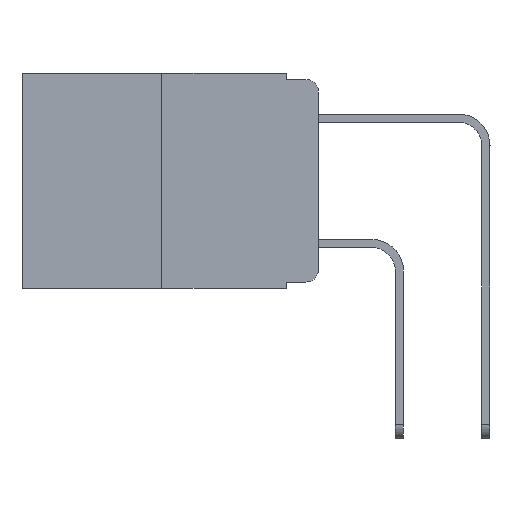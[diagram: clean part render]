
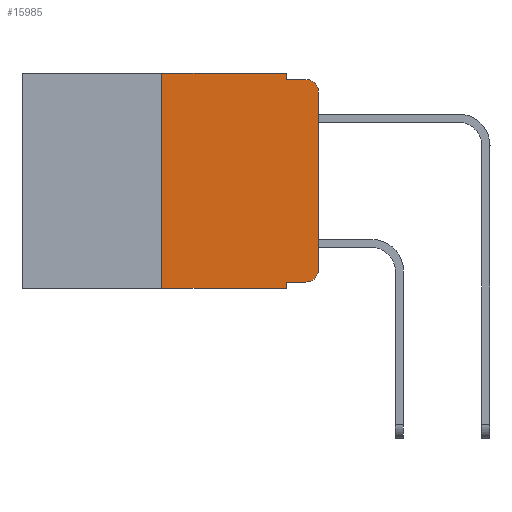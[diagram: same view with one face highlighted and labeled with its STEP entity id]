
A CAD part, left-side view. The second image highlights one B-rep face of the part: STEP entity #15985.
In plain terms, the highlighted planar face has unit normal (-1, 0, 0).
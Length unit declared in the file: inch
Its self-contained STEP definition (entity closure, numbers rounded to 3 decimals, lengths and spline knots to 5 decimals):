
#83 = VECTOR ( 'NONE', #18770, 39.37008 ) ;
#1247 = DIRECTION ( 'NONE',  ( 0., -1., 0. ) ) ;
#1356 = EDGE_CURVE ( 'NONE', #2703, #6175, #15612, .T. ) ;
#1465 = PLANE ( 'NONE',  #12127 ) ;
#1595 = EDGE_CURVE ( 'NONE', #11522, #7091, #17260, .T. ) ;
#1651 = CARTESIAN_POINT ( 'NONE',  ( 0., 0.051, -0.01 ) ) ;
#1999 = EDGE_CURVE ( 'NONE', #16640, #8751, #3684, .T. ) ;
#2165 = ORIENTED_EDGE ( 'NONE', *, *, #15334, .T. ) ;
#2244 = CARTESIAN_POINT ( 'NONE',  ( 0., 0., 0. ) ) ;
#2339 = ORIENTED_EDGE ( 'NONE', *, *, #1595, .F. ) ;
#2703 = VERTEX_POINT ( 'NONE', #9197 ) ;
#3211 = ORIENTED_EDGE ( 'NONE', *, *, #10394, .F. ) ;
#3255 = AXIS2_PLACEMENT_3D ( 'NONE', #13335, #4582, #4142 ) ;
#3684 = CIRCLE ( 'NONE', #13713, 0.02 ) ;
#3781 = VECTOR ( 'NONE', #10715, 39.37008 ) ;
#3788 = LINE ( 'NONE', #1651, #3781 ) ;
#3807 = DIRECTION ( 'NONE',  ( 0., -1., 0. ) ) ;
#3829 = DIRECTION ( 'NONE',  ( 0., 0., -1. ) ) ;
#4125 = FACE_OUTER_BOUND ( 'NONE', #10324, .T. ) ;
#4142 = DIRECTION ( 'NONE',  ( 0., 0., -1. ) ) ;
#4145 = LINE ( 'NONE', #5860, #5555 ) ;
#4582 = DIRECTION ( 'NONE',  ( -1., 0., 0. ) ) ;
#4693 = LINE ( 'NONE', #7018, #19431 ) ;
#5419 = EDGE_CURVE ( 'NONE', #13062, #10968, #4693, .T. ) ;
#5555 = VECTOR ( 'NONE', #10460, 39.37008 ) ;
#5860 = CARTESIAN_POINT ( 'NONE',  ( 0., 0.051, -0.333 ) ) ;
#6067 = CARTESIAN_POINT ( 'NONE',  ( 0., 0.473, 0. ) ) ;
#6175 = VERTEX_POINT ( 'NONE', #8350 ) ;
#6269 = CIRCLE ( 'NONE', #3255, 0.02 ) ;
#6713 = LINE ( 'NONE', #15894, #13593 ) ;
#7018 = CARTESIAN_POINT ( 'NONE',  ( 0., 0.051, 0. ) ) ;
#7091 = VERTEX_POINT ( 'NONE', #19021 ) ;
#7314 = DIRECTION ( 'NONE',  ( 0., 0., -1. ) ) ;
#7614 = DIRECTION ( 'NONE',  ( 0., 0., -1. ) ) ;
#7619 = DIRECTION ( 'NONE',  ( 0., 0., -1. ) ) ;
#7679 = DIRECTION ( 'NONE',  ( -1., 0., 0. ) ) ;
#7975 = VERTEX_POINT ( 'NONE', #14895 ) ;
#8350 = CARTESIAN_POINT ( 'NONE',  ( 0., 0.25, 0. ) ) ;
#8414 = CARTESIAN_POINT ( 'NONE',  ( 0., 0.051, 0. ) ) ;
#8751 = VERTEX_POINT ( 'NONE', #10930 ) ;
#9197 = CARTESIAN_POINT ( 'NONE',  ( 0., 0.25, -0.343 ) ) ;
#9315 = CARTESIAN_POINT ( 'NONE',  ( 0., 0.051, -0.01 ) ) ;
#9474 = ORIENTED_EDGE ( 'NONE', *, *, #10550, .T. ) ;
#9818 = ORIENTED_EDGE ( 'NONE', *, *, #16321, .T. ) ;
#10324 = EDGE_LOOP ( 'NONE', ( #9818, #11984, #10489, #15270, #3211, #14502, #9474, #2339, #2165, #16819 ) ) ;
#10394 = EDGE_CURVE ( 'NONE', #6175, #13062, #16227, .T. ) ;
#10460 = DIRECTION ( 'NONE',  ( 0., -1., 0. ) ) ;
#10489 = ORIENTED_EDGE ( 'NONE', *, *, #12215, .F. ) ;
#10550 = EDGE_CURVE ( 'NONE', #2703, #7091, #6713, .T. ) ;
#10715 = DIRECTION ( 'NONE',  ( 0., -1., 0. ) ) ;
#10930 = CARTESIAN_POINT ( 'NONE',  ( 0., 0., -0.313 ) ) ;
#10968 = VERTEX_POINT ( 'NONE', #9315 ) ;
#11522 = VERTEX_POINT ( 'NONE', #16805 ) ;
#11984 = ORIENTED_EDGE ( 'NONE', *, *, #15957, .T. ) ;
#12042 = DIRECTION ( 'NONE',  ( 1., 0., 0. ) ) ;
#12127 = AXIS2_PLACEMENT_3D ( 'NONE', #16720, #12042, #7614 ) ;
#12215 = EDGE_CURVE ( 'NONE', #10968, #7975, #3788, .T. ) ;
#12397 = CARTESIAN_POINT ( 'NONE',  ( 0., 0.25, 0. ) ) ;
#13062 = VERTEX_POINT ( 'NONE', #8414 ) ;
#13335 = CARTESIAN_POINT ( 'NONE',  ( 0., 0.02, -0.03 ) ) ;
#13593 = VECTOR ( 'NONE', #3807, 39.37008 ) ;
#13713 = AXIS2_PLACEMENT_3D ( 'NONE', #16724, #7679, #7619 ) ;
#13939 = DIRECTION ( 'NONE',  ( 0., 0., 1. ) ) ;
#14413 = VERTEX_POINT ( 'NONE', #18862 ) ;
#14502 = ORIENTED_EDGE ( 'NONE', *, *, #1356, .F. ) ;
#14895 = CARTESIAN_POINT ( 'NONE',  ( 0., 0.02, -0.01 ) ) ;
#15270 = ORIENTED_EDGE ( 'NONE', *, *, #5419, .F. ) ;
#15334 = EDGE_CURVE ( 'NONE', #11522, #16640, #4145, .T. ) ;
#15612 = LINE ( 'NONE', #12397, #16317 ) ;
#15894 = CARTESIAN_POINT ( 'NONE',  ( 0., 0.473, -0.343 ) ) ;
#15957 = EDGE_CURVE ( 'NONE', #14413, #7975, #6269, .T. ) ;
#15985 = ADVANCED_FACE ( 'NONE', ( #4125 ), #1465, .F. ) ;
#16227 = LINE ( 'NONE', #6067, #17900 ) ;
#16279 = CARTESIAN_POINT ( 'NONE',  ( 0., 0.051, 0. ) ) ;
#16317 = VECTOR ( 'NONE', #13939, 39.37008 ) ;
#16321 = EDGE_CURVE ( 'NONE', #8751, #14413, #16719, .T. ) ;
#16640 = VERTEX_POINT ( 'NONE', #18238 ) ;
#16719 = LINE ( 'NONE', #2244, #83 ) ;
#16720 = CARTESIAN_POINT ( 'NONE',  ( 0., 0.473, 0. ) ) ;
#16724 = CARTESIAN_POINT ( 'NONE',  ( 0., 0.02, -0.313 ) ) ;
#16805 = CARTESIAN_POINT ( 'NONE',  ( 0., 0.051, -0.333 ) ) ;
#16819 = ORIENTED_EDGE ( 'NONE', *, *, #1999, .T. ) ;
#17260 = LINE ( 'NONE', #16279, #18924 ) ;
#17900 = VECTOR ( 'NONE', #1247, 39.37008 ) ;
#18238 = CARTESIAN_POINT ( 'NONE',  ( 0., 0.02, -0.333 ) ) ;
#18770 = DIRECTION ( 'NONE',  ( 0., 0., 1. ) ) ;
#18862 = CARTESIAN_POINT ( 'NONE',  ( 0., 0., -0.03 ) ) ;
#18924 = VECTOR ( 'NONE', #7314, 39.37008 ) ;
#19021 = CARTESIAN_POINT ( 'NONE',  ( 0., 0.051, -0.343 ) ) ;
#19431 = VECTOR ( 'NONE', #3829, 39.37008 ) ;
